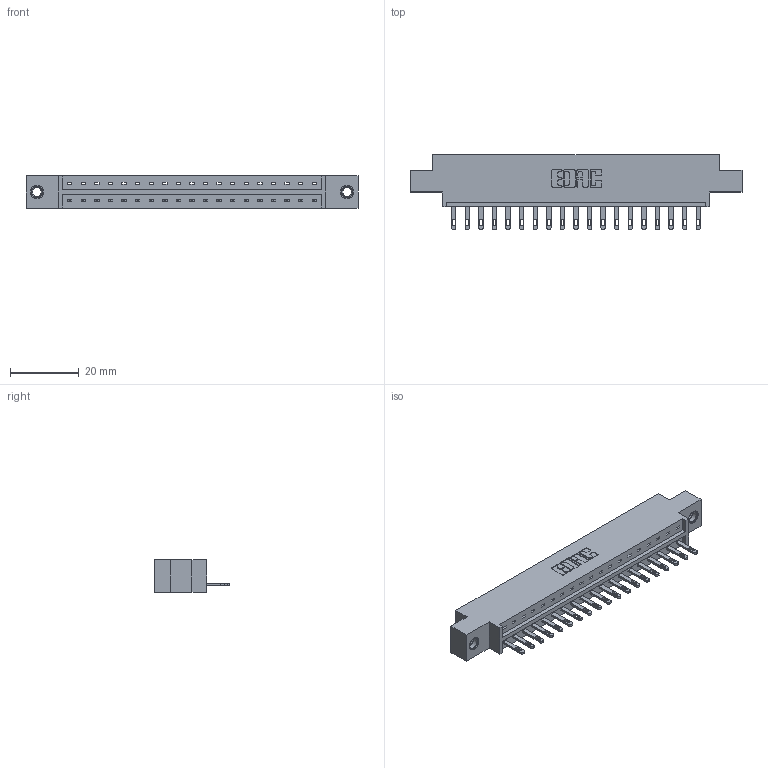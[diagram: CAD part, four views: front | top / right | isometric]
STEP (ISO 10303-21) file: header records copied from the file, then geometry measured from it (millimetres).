
FILE_DESCRIPTION (( 'STEP AP203' ), '1' );
FILE_NAME ('833-019-500-607.STEP', '2020-05-31T23:51:10', ( '' ), ( '' ), 'SwSTEP 2.0', 'SolidWorks 2020', '' );
FILE_SCHEMA (( 'CONFIG_CONTROL_DESIGN' ));
Length unit declared in the file: inch
Products named in the file (4): 345-250-001_345-250-005-103; 833 Part_Offset - .156 Dia - TI; 345-292-001_345-293-100; 833-019-500-607
Assembly tree (22 placements, depth 2):
  833-019-500-607
    833 Part_Offset - .156 Dia - TI
    345-292-001_345-293-100  x19
    345-250-001_345-250-005-103  x2
Bounding box: 96.82 x 21.85 x 9.4 mm (x, y, z)
Volume: 9316 mm3; surface area: 10210.8 mm2
Topology: 22 solids, 22 shells, 1204 faces, 3651 edges, 2426 vertices
Faces by surface type: plane 790, cylinder 398, cone 12, torus 4
Entity records: 15838 total; most frequent: CARTESIAN_POINT 2718, ORIENTED_EDGE 2666, DIRECTION 2373, EDGE_CURVE 1333, LINE 1181, VECTOR 1181, VERTEX_POINT 884, AXIS2_PLACEMENT_3D 596
